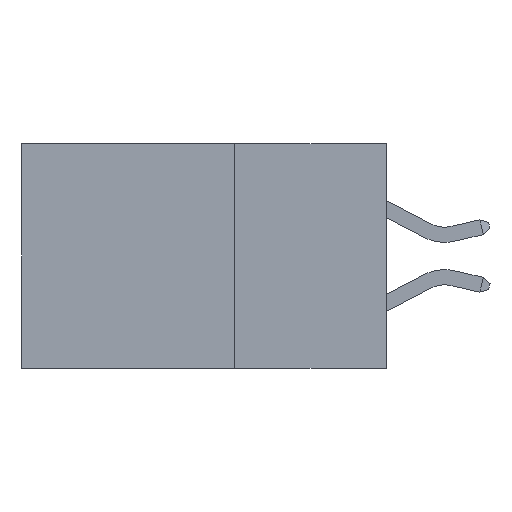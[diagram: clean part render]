
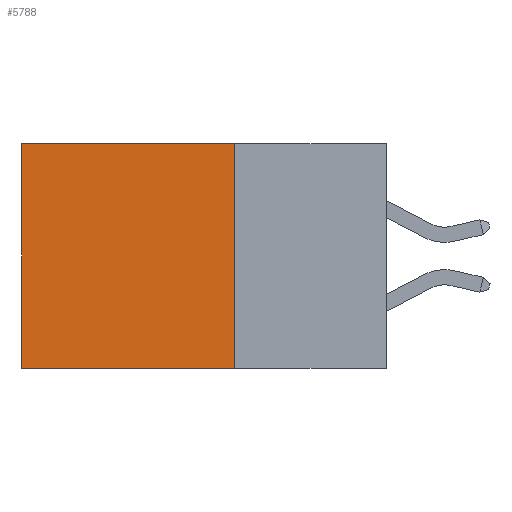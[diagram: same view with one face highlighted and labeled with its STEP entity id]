
A CAD part, left-side view. The second image highlights one B-rep face of the part: STEP entity #5788.
In plain terms, the highlighted planar face has unit normal (-1, 0, 0).
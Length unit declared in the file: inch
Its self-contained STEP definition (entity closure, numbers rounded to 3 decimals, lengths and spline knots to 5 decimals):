
#3732 = CARTESIAN_POINT ( 'NONE',  ( 0.298, 0.6, -0.37 ) ) ;
#4164 = EDGE_CURVE ( 'NONE', #21945, #11959, #30938, .T. ) ;
#5098 = CARTESIAN_POINT ( 'NONE',  ( 0.298, 0.25, 0. ) ) ;
#5232 = VECTOR ( 'NONE', #11890, 39.37008 ) ;
#5513 = VECTOR ( 'NONE', #9295, 39.37008 ) ;
#5788 = ADVANCED_FACE ( 'NONE', ( #18329 ), #23852, .F. ) ;
#6557 = ORIENTED_EDGE ( 'NONE', *, *, #18588, .F. ) ;
#9093 = EDGE_CURVE ( 'NONE', #15650, #29988, #11693, .T. ) ;
#9295 = DIRECTION ( 'NONE',  ( 0., 0., -1. ) ) ;
#10332 = ORIENTED_EDGE ( 'NONE', *, *, #9093, .T. ) ;
#10748 = CARTESIAN_POINT ( 'NONE',  ( 0.298, 0.25, -0.37 ) ) ;
#11693 = LINE ( 'NONE', #21743, #5232 ) ;
#11890 = DIRECTION ( 'NONE',  ( 0., 1., 0. ) ) ;
#11959 = VERTEX_POINT ( 'NONE', #3732 ) ;
#11977 = CARTESIAN_POINT ( 'NONE',  ( 0.298, 0.25, -0.37 ) ) ;
#14853 = DIRECTION ( 'NONE',  ( 0., 0., -1. ) ) ;
#15650 = VERTEX_POINT ( 'NONE', #5098 ) ;
#18329 = FACE_OUTER_BOUND ( 'NONE', #29392, .T. ) ;
#18588 = EDGE_CURVE ( 'NONE', #15650, #21945, #24877, .T. ) ;
#19292 = ORIENTED_EDGE ( 'NONE', *, *, #4164, .F. ) ;
#19394 = CARTESIAN_POINT ( 'NONE',  ( 0.298, 0.6, 0. ) ) ;
#19613 = DIRECTION ( 'NONE',  ( 1., 0., 0. ) ) ;
#20698 = DIRECTION ( 'NONE',  ( 0., 1., 0. ) ) ;
#21590 = AXIS2_PLACEMENT_3D ( 'NONE', #29363, #19613, #14853 ) ;
#21743 = CARTESIAN_POINT ( 'NONE',  ( 0.298, 0.25, 0. ) ) ;
#21945 = VERTEX_POINT ( 'NONE', #11977 ) ;
#22536 = EDGE_CURVE ( 'NONE', #29988, #11959, #31299, .T. ) ;
#23720 = VECTOR ( 'NONE', #20698, 39.37008 ) ;
#23819 = CARTESIAN_POINT ( 'NONE',  ( 0.298, 0.6, 0. ) ) ;
#23852 = PLANE ( 'NONE',  #21590 ) ;
#24877 = LINE ( 'NONE', #26234, #30215 ) ;
#25526 = ORIENTED_EDGE ( 'NONE', *, *, #22536, .T. ) ;
#26234 = CARTESIAN_POINT ( 'NONE',  ( 0.298, 0.25, 0. ) ) ;
#29363 = CARTESIAN_POINT ( 'NONE',  ( 0.298, 0.25, 0. ) ) ;
#29392 = EDGE_LOOP ( 'NONE', ( #25526, #19292, #6557, #10332 ) ) ;
#29988 = VERTEX_POINT ( 'NONE', #19394 ) ;
#30215 = VECTOR ( 'NONE', #30375, 39.37008 ) ;
#30375 = DIRECTION ( 'NONE',  ( 0., 0., -1. ) ) ;
#30938 = LINE ( 'NONE', #10748, #23720 ) ;
#31299 = LINE ( 'NONE', #23819, #5513 ) ;
